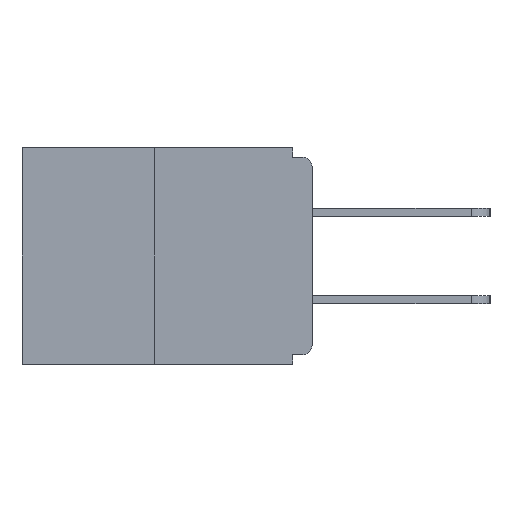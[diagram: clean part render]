
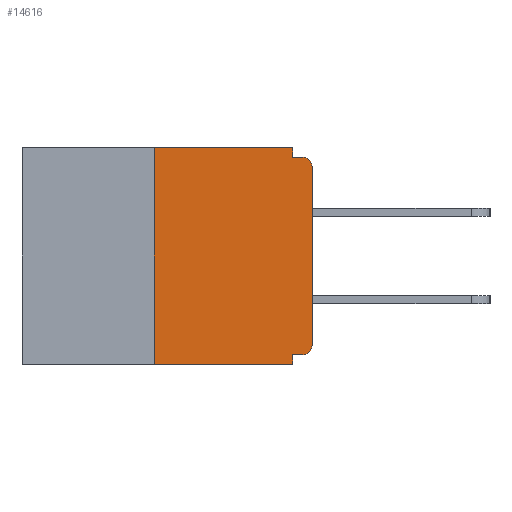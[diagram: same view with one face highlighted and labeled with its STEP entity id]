
A CAD part, left-side view. The second image highlights one B-rep face of the part: STEP entity #14616.
In plain terms, the highlighted planar face has unit normal (-1, 0, 0).
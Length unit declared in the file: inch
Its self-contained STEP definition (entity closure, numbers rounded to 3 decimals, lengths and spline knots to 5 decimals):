
#671 = CARTESIAN_POINT ( 'NONE',  ( 0., 0.031, 0. ) ) ;
#917 = LINE ( 'NONE', #19803, #18026 ) ;
#1207 = CARTESIAN_POINT ( 'NONE',  ( 0., 0., -0.03 ) ) ;
#1527 = DIRECTION ( 'NONE',  ( 0., 0., -1. ) ) ;
#1654 = VECTOR ( 'NONE', #14325, 39.37008 ) ;
#1872 = EDGE_CURVE ( 'NONE', #17849, #14778, #6356, .T. ) ;
#2286 = AXIS2_PLACEMENT_3D ( 'NONE', #12792, #11044, #3145 ) ;
#2615 = ORIENTED_EDGE ( 'NONE', *, *, #12459, .T. ) ;
#2692 = CARTESIAN_POINT ( 'NONE',  ( 0., 0.46, 0. ) ) ;
#3101 = CARTESIAN_POINT ( 'NONE',  ( 0., 0.031, -0.343 ) ) ;
#3145 = DIRECTION ( 'NONE',  ( 0., 0., -1. ) ) ;
#3699 = VERTEX_POINT ( 'NONE', #17501 ) ;
#4251 = VECTOR ( 'NONE', #17560, 39.37008 ) ;
#4390 = VECTOR ( 'NONE', #7509, 39.37008 ) ;
#4517 = CARTESIAN_POINT ( 'NONE',  ( 0., 0., -0.015 ) ) ;
#4976 = EDGE_CURVE ( 'NONE', #8879, #11262, #5182, .T. ) ;
#5182 = LINE ( 'NONE', #20140, #7218 ) ;
#5230 = LINE ( 'NONE', #4517, #4251 ) ;
#5902 = LINE ( 'NONE', #7422, #20871 ) ;
#5922 = LINE ( 'NONE', #7888, #1654 ) ;
#6261 = CARTESIAN_POINT ( 'NONE',  ( 0., 0.031, -0.343 ) ) ;
#6356 = CIRCLE ( 'NONE', #2286, 0.015 ) ;
#6529 = CARTESIAN_POINT ( 'NONE',  ( 0., 0.015, -0.015 ) ) ;
#6715 = CARTESIAN_POINT ( 'NONE',  ( 0., 0.015, -0.328 ) ) ;
#7218 = VECTOR ( 'NONE', #15135, 39.37008 ) ;
#7422 = CARTESIAN_POINT ( 'NONE',  ( 0., 0., 0. ) ) ;
#7509 = DIRECTION ( 'NONE',  ( 0., 0., 1. ) ) ;
#7544 = DIRECTION ( 'NONE',  ( -1., 0., 0. ) ) ;
#7888 = CARTESIAN_POINT ( 'NONE',  ( 0., 0., -0.328 ) ) ;
#8210 = ORIENTED_EDGE ( 'NONE', *, *, #20801, .F. ) ;
#8429 = EDGE_CURVE ( 'NONE', #19926, #12847, #17513, .T. ) ;
#8649 = CARTESIAN_POINT ( 'NONE',  ( 0., 0.031, 0. ) ) ;
#8879 = VERTEX_POINT ( 'NONE', #16258 ) ;
#8994 = CARTESIAN_POINT ( 'NONE',  ( 0., 0.031, -0.328 ) ) ;
#9114 = ORIENTED_EDGE ( 'NONE', *, *, #14168, .F. ) ;
#9278 = ORIENTED_EDGE ( 'NONE', *, *, #10736, .F. ) ;
#10221 = AXIS2_PLACEMENT_3D ( 'NONE', #17234, #7544, #18876 ) ;
#10345 = ORIENTED_EDGE ( 'NONE', *, *, #12092, .F. ) ;
#10581 = PLANE ( 'NONE',  #11699 ) ;
#10736 = EDGE_CURVE ( 'NONE', #18476, #12847, #5230, .T. ) ;
#10741 = DIRECTION ( 'NONE',  ( 0., 0., 1. ) ) ;
#10917 = VECTOR ( 'NONE', #18426, 39.37008 ) ;
#11044 = DIRECTION ( 'NONE',  ( -1., 0., 0. ) ) ;
#11262 = VERTEX_POINT ( 'NONE', #671 ) ;
#11699 = AXIS2_PLACEMENT_3D ( 'NONE', #2692, #12057, #18805 ) ;
#11943 = LINE ( 'NONE', #20693, #4390 ) ;
#12057 = DIRECTION ( 'NONE',  ( 1., 0., 0. ) ) ;
#12092 = EDGE_CURVE ( 'NONE', #17849, #18193, #5922, .T. ) ;
#12405 = EDGE_LOOP ( 'NONE', ( #16184, #16743, #14078, #9114, #10345, #16879, #2615, #13307, #9278, #8210 ) ) ;
#12459 = EDGE_CURVE ( 'NONE', #14778, #19926, #5902, .T. ) ;
#12792 = CARTESIAN_POINT ( 'NONE',  ( 0., 0.015, -0.313 ) ) ;
#12847 = VERTEX_POINT ( 'NONE', #6529 ) ;
#13111 = FACE_OUTER_BOUND ( 'NONE', #12405, .T. ) ;
#13307 = ORIENTED_EDGE ( 'NONE', *, *, #8429, .T. ) ;
#13450 = EDGE_CURVE ( 'NONE', #3699, #8879, #11943, .T. ) ;
#13674 = VECTOR ( 'NONE', #1527, 39.37008 ) ;
#13713 = LINE ( 'NONE', #8649, #10917 ) ;
#13936 = LINE ( 'NONE', #6261, #13674 ) ;
#14078 = ORIENTED_EDGE ( 'NONE', *, *, #20070, .T. ) ;
#14168 = EDGE_CURVE ( 'NONE', #18193, #17148, #13936, .T. ) ;
#14325 = DIRECTION ( 'NONE',  ( 0., 1., 0. ) ) ;
#14370 = CARTESIAN_POINT ( 'NONE',  ( 0., 0., -0.313 ) ) ;
#14616 = ADVANCED_FACE ( 'NONE', ( #13111 ), #10581, .F. ) ;
#14778 = VERTEX_POINT ( 'NONE', #14370 ) ;
#15093 = DIRECTION ( 'NONE',  ( 0., -1., 0. ) ) ;
#15135 = DIRECTION ( 'NONE',  ( 0., -1., 0. ) ) ;
#16184 = ORIENTED_EDGE ( 'NONE', *, *, #4976, .F. ) ;
#16196 = CARTESIAN_POINT ( 'NONE',  ( 0., 0.031, -0.015 ) ) ;
#16258 = CARTESIAN_POINT ( 'NONE',  ( 0., 0.25, 0. ) ) ;
#16743 = ORIENTED_EDGE ( 'NONE', *, *, #13450, .F. ) ;
#16879 = ORIENTED_EDGE ( 'NONE', *, *, #1872, .T. ) ;
#17148 = VERTEX_POINT ( 'NONE', #3101 ) ;
#17234 = CARTESIAN_POINT ( 'NONE',  ( 0., 0.015, -0.03 ) ) ;
#17501 = CARTESIAN_POINT ( 'NONE',  ( 0., 0.25, -0.343 ) ) ;
#17513 = CIRCLE ( 'NONE', #10221, 0.015 ) ;
#17560 = DIRECTION ( 'NONE',  ( 0., -1., 0. ) ) ;
#17849 = VERTEX_POINT ( 'NONE', #6715 ) ;
#18026 = VECTOR ( 'NONE', #15093, 39.37008 ) ;
#18193 = VERTEX_POINT ( 'NONE', #8994 ) ;
#18426 = DIRECTION ( 'NONE',  ( 0., 0., -1. ) ) ;
#18476 = VERTEX_POINT ( 'NONE', #16196 ) ;
#18805 = DIRECTION ( 'NONE',  ( 0., 0., -1. ) ) ;
#18876 = DIRECTION ( 'NONE',  ( 0., 0., -1. ) ) ;
#19803 = CARTESIAN_POINT ( 'NONE',  ( 0., 0.46, -0.343 ) ) ;
#19926 = VERTEX_POINT ( 'NONE', #1207 ) ;
#20070 = EDGE_CURVE ( 'NONE', #3699, #17148, #917, .T. ) ;
#20140 = CARTESIAN_POINT ( 'NONE',  ( 0., 0.46, 0. ) ) ;
#20693 = CARTESIAN_POINT ( 'NONE',  ( 0., 0.25, 0. ) ) ;
#20801 = EDGE_CURVE ( 'NONE', #11262, #18476, #13713, .T. ) ;
#20871 = VECTOR ( 'NONE', #10741, 39.37008 ) ;
